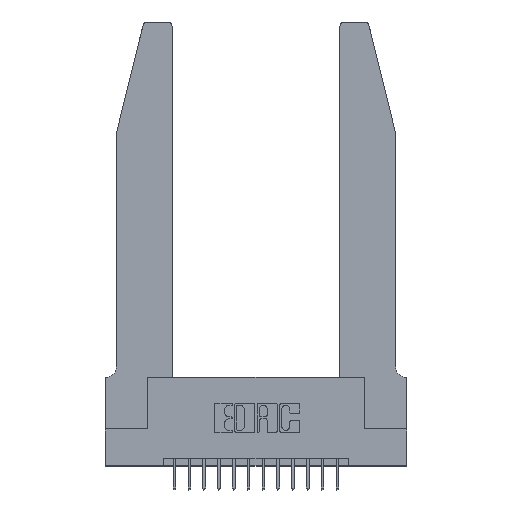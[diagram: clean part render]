
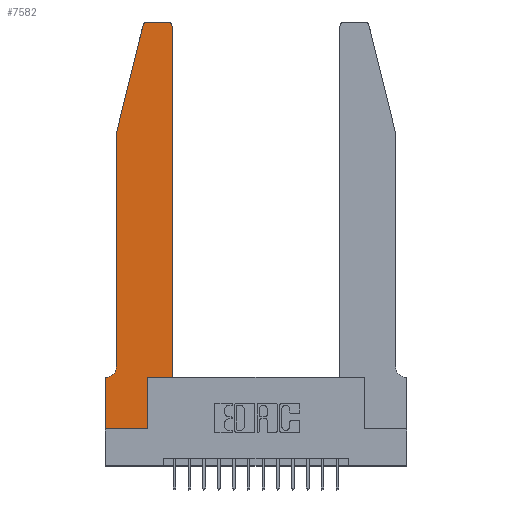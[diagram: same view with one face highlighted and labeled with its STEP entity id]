
A CAD part, top view. The second image highlights one B-rep face of the part: STEP entity #7582.
In plain terms, the highlighted planar face has unit normal (0, 0, 1).
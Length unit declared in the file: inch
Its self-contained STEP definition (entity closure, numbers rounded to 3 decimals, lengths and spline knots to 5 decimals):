
#16 = VECTOR ( 'NONE', #13004, 39.37008 ) ;
#452 = CARTESIAN_POINT ( 'NONE',  ( 0.4505, 0.35, 0.37 ) ) ;
#611 = VERTEX_POINT ( 'NONE', #10012 ) ;
#813 = CARTESIAN_POINT ( 'NONE',  ( 0.4505, 0.35, 0.37 ) ) ;
#1319 = ORIENTED_EDGE ( 'NONE', *, *, #12758, .T. ) ;
#1554 = CARTESIAN_POINT ( 'NONE',  ( 0.284, 2.75, 0.37 ) ) ;
#1569 = CARTESIAN_POINT ( 'NONE',  ( 0.4205, 2.75, 0.37 ) ) ;
#1665 = EDGE_CURVE ( 'NONE', #3742, #3442, #6875, .T. ) ;
#1678 = AXIS2_PLACEMENT_3D ( 'NONE', #3043, #12960, #4559 ) ;
#2229 = CIRCLE ( 'NONE', #5109, 0.03 ) ;
#2657 = VERTEX_POINT ( 'NONE', #12492 ) ;
#2786 = EDGE_CURVE ( 'NONE', #611, #6622, #7818, .T. ) ;
#2895 = LINE ( 'NONE', #813, #17278 ) ;
#2908 = DIRECTION ( 'NONE',  ( 0., -1., 0. ) ) ;
#3033 = ORIENTED_EDGE ( 'NONE', *, *, #12598, .T. ) ;
#3043 = CARTESIAN_POINT ( 'NONE',  ( 0.0055, 0.42, 0.37 ) ) ;
#3350 = ORIENTED_EDGE ( 'NONE', *, *, #9607, .T. ) ;
#3414 = CARTESIAN_POINT ( 'NONE',  ( 0.4505, 0.35, 0.37 ) ) ;
#3442 = VERTEX_POINT ( 'NONE', #1554 ) ;
#3742 = VERTEX_POINT ( 'NONE', #1569 ) ;
#3930 = CIRCLE ( 'NONE', #14076, 0.03 ) ;
#4023 = ORIENTED_EDGE ( 'NONE', *, *, #5511, .T. ) ;
#4119 = LINE ( 'NONE', #17819, #6586 ) ;
#4559 = DIRECTION ( 'NONE',  ( -1., 0., 0. ) ) ;
#4580 = DIRECTION ( 'NONE',  ( -1., 0., 0. ) ) ;
#4685 = VERTEX_POINT ( 'NONE', #5239 ) ;
#4729 = ORIENTED_EDGE ( 'NONE', *, *, #15295, .T. ) ;
#4977 = VERTEX_POINT ( 'NONE', #5973 ) ;
#5058 = VECTOR ( 'NONE', #2908, 39.37008 ) ;
#5109 = AXIS2_PLACEMENT_3D ( 'NONE', #8155, #17654, #9583 ) ;
#5239 = CARTESIAN_POINT ( 'NONE',  ( 0., 0.35, 0.37 ) ) ;
#5458 = DIRECTION ( 'NONE',  ( 0., 0., 1. ) ) ;
#5511 = EDGE_CURVE ( 'NONE', #4685, #611, #8847, .T. ) ;
#5515 = DIRECTION ( 'NONE',  ( 0., 0., 1. ) ) ;
#5559 = ORIENTED_EDGE ( 'NONE', *, *, #2786, .T. ) ;
#5587 = EDGE_CURVE ( 'NONE', #9751, #4685, #15247, .T. ) ;
#5793 = DIRECTION ( 'NONE',  ( 0., -1., 0. ) ) ;
#5799 = VECTOR ( 'NONE', #9162, 39.37008 ) ;
#5973 = CARTESIAN_POINT ( 'NONE',  ( 0.2865, 0.35, 0.37 ) ) ;
#6530 = ORIENTED_EDGE ( 'NONE', *, *, #5587, .T. ) ;
#6586 = VECTOR ( 'NONE', #8323, 39.37008 ) ;
#6622 = VERTEX_POINT ( 'NONE', #13850 ) ;
#6875 = LINE ( 'NONE', #10849, #14223 ) ;
#6888 = EDGE_CURVE ( 'NONE', #12917, #2657, #2895, .T. ) ;
#7435 = FACE_OUTER_BOUND ( 'NONE', #15843, .T. ) ;
#7582 = ADVANCED_FACE ( 'NONE', ( #7435 ), #9739, .T. ) ;
#7818 = LINE ( 'NONE', #14012, #8715 ) ;
#8155 = CARTESIAN_POINT ( 'NONE',  ( 0.4205, 2.72, 0.37 ) ) ;
#8185 = CARTESIAN_POINT ( 'NONE',  ( 0.0055, 0.35, 0.37 ) ) ;
#8309 = CARTESIAN_POINT ( 'NONE',  ( 0., 0.35, 0.37 ) ) ;
#8323 = DIRECTION ( 'NONE',  ( -0.239, -0.971, 0. ) ) ;
#8682 = DIRECTION ( 'NONE',  ( 1., 0., 0. ) ) ;
#8715 = VECTOR ( 'NONE', #8682, 39.37008 ) ;
#8847 = LINE ( 'NONE', #11470, #5058 ) ;
#9162 = DIRECTION ( 'NONE',  ( 0., 1., 0. ) ) ;
#9377 = ORIENTED_EDGE ( 'NONE', *, *, #15082, .T. ) ;
#9583 = DIRECTION ( 'NONE',  ( 1., 0., 0. ) ) ;
#9607 = EDGE_CURVE ( 'NONE', #4977, #12917, #11175, .T. ) ;
#9739 = PLANE ( 'NONE',  #16144 ) ;
#9751 = VERTEX_POINT ( 'NONE', #8185 ) ;
#10012 = CARTESIAN_POINT ( 'NONE',  ( 0., 0., 0.37 ) ) ;
#10379 = CARTESIAN_POINT ( 'NONE',  ( 0.25487, 2.72718, 0.37 ) ) ;
#10436 = ORIENTED_EDGE ( 'NONE', *, *, #15860, .T. ) ;
#10555 = CIRCLE ( 'NONE', #1678, 0.07 ) ;
#10849 = CARTESIAN_POINT ( 'NONE',  ( 0.2605, 2.75, 0.37 ) ) ;
#11058 = LINE ( 'NONE', #14085, #11898 ) ;
#11085 = DIRECTION ( 'NONE',  ( 0., 1., 0. ) ) ;
#11175 = LINE ( 'NONE', #452, #13908 ) ;
#11470 = CARTESIAN_POINT ( 'NONE',  ( 0., 0., 0.37 ) ) ;
#11640 = CARTESIAN_POINT ( 'NONE',  ( 0.0755, 0.35, 0.37 ) ) ;
#11898 = VECTOR ( 'NONE', #5793, 39.37008 ) ;
#12079 = DIRECTION ( 'NONE',  ( 1., 0., 0. ) ) ;
#12147 = ORIENTED_EDGE ( 'NONE', *, *, #6888, .T. ) ;
#12398 = VERTEX_POINT ( 'NONE', #10379 ) ;
#12492 = CARTESIAN_POINT ( 'NONE',  ( 0.4505, 2.72, 0.37 ) ) ;
#12522 = CARTESIAN_POINT ( 'NONE',  ( 0.0755, 2., 0.37 ) ) ;
#12598 = EDGE_CURVE ( 'NONE', #2657, #3742, #2229, .T. ) ;
#12758 = EDGE_CURVE ( 'NONE', #16161, #13771, #11058, .T. ) ;
#12917 = VERTEX_POINT ( 'NONE', #3414 ) ;
#12960 = DIRECTION ( 'NONE',  ( 0., 0., -1. ) ) ;
#13004 = DIRECTION ( 'NONE',  ( -1., 0., 0. ) ) ;
#13151 = EDGE_CURVE ( 'NONE', #3442, #12398, #3930, .T. ) ;
#13199 = ORIENTED_EDGE ( 'NONE', *, *, #1665, .T. ) ;
#13771 = VERTEX_POINT ( 'NONE', #16284 ) ;
#13789 = CARTESIAN_POINT ( 'NONE',  ( 0.284, 2.72, 0.37 ) ) ;
#13850 = CARTESIAN_POINT ( 'NONE',  ( 0.2865, 0., 0.37 ) ) ;
#13908 = VECTOR ( 'NONE', #12079, 39.37008 ) ;
#14012 = CARTESIAN_POINT ( 'NONE',  ( 0., 0., 0.37 ) ) ;
#14076 = AXIS2_PLACEMENT_3D ( 'NONE', #13789, #5458, #15143 ) ;
#14085 = CARTESIAN_POINT ( 'NONE',  ( 0.0755, 2., 0.37 ) ) ;
#14223 = VECTOR ( 'NONE', #4580, 39.37008 ) ;
#15082 = EDGE_CURVE ( 'NONE', #12398, #16161, #4119, .T. ) ;
#15143 = DIRECTION ( 'NONE',  ( 1., 0., 0. ) ) ;
#15189 = DIRECTION ( 'NONE',  ( 1., 0., 0. ) ) ;
#15247 = LINE ( 'NONE', #11640, #16 ) ;
#15295 = EDGE_CURVE ( 'NONE', #13771, #9751, #10555, .T. ) ;
#15843 = EDGE_LOOP ( 'NONE', ( #13199, #17607, #9377, #1319, #4729, #6530, #4023, #5559, #10436, #3350, #12147, #3033 ) ) ;
#15860 = EDGE_CURVE ( 'NONE', #6622, #4977, #16336, .T. ) ;
#16144 = AXIS2_PLACEMENT_3D ( 'NONE', #8309, #5515, #15189 ) ;
#16161 = VERTEX_POINT ( 'NONE', #12522 ) ;
#16284 = CARTESIAN_POINT ( 'NONE',  ( 0.0755, 0.42, 0.37 ) ) ;
#16336 = LINE ( 'NONE', #17261, #5799 ) ;
#17261 = CARTESIAN_POINT ( 'NONE',  ( 0.2865, 0.35, 0.37 ) ) ;
#17278 = VECTOR ( 'NONE', #11085, 39.37008 ) ;
#17607 = ORIENTED_EDGE ( 'NONE', *, *, #13151, .T. ) ;
#17654 = DIRECTION ( 'NONE',  ( 0., 0., 1. ) ) ;
#17819 = CARTESIAN_POINT ( 'NONE',  ( 0.0755, 2., 0.37 ) ) ;
